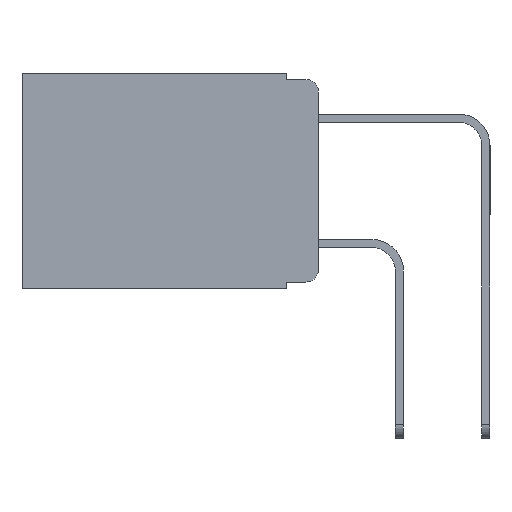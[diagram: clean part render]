
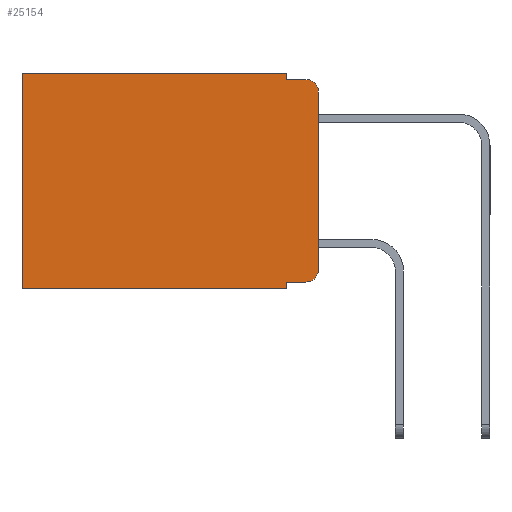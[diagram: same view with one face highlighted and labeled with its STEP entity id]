
A CAD part, left-side view. The second image highlights one B-rep face of the part: STEP entity #25154.
In plain terms, the highlighted planar face has unit normal (-1, 0, 0).
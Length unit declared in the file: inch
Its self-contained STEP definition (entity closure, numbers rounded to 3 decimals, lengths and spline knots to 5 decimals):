
#97 = CARTESIAN_POINT ( 'NONE',  ( 0.298, 0.02, -0.333 ) ) ;
#157 = ORIENTED_EDGE ( 'NONE', *, *, #8219, .T. ) ;
#265 = LINE ( 'NONE', #22726, #15588 ) ;
#322 = DIRECTION ( 'NONE',  ( 0., 0., -1. ) ) ;
#999 = EDGE_CURVE ( 'NONE', #4559, #19389, #6446, .T. ) ;
#1162 = CARTESIAN_POINT ( 'NONE',  ( 0.298, 0.051, 0. ) ) ;
#1246 = DIRECTION ( 'NONE',  ( 0., 0., -1. ) ) ;
#1251 = CARTESIAN_POINT ( 'NONE',  ( 0.298, 0.051, -0.01 ) ) ;
#2074 = VECTOR ( 'NONE', #15118, 39.37008 ) ;
#3204 = CARTESIAN_POINT ( 'NONE',  ( 0.298, 0.473, 0. ) ) ;
#3210 = DIRECTION ( 'NONE',  ( 0., 0., -1. ) ) ;
#3234 = CARTESIAN_POINT ( 'NONE',  ( 0.298, 0., -0.313 ) ) ;
#3296 = DIRECTION ( 'NONE',  ( 0., -1., 0. ) ) ;
#3695 = ORIENTED_EDGE ( 'NONE', *, *, #11364, .F. ) ;
#3890 = ORIENTED_EDGE ( 'NONE', *, *, #19083, .F. ) ;
#4059 = ORIENTED_EDGE ( 'NONE', *, *, #4379, .T. ) ;
#4379 = EDGE_CURVE ( 'NONE', #19259, #4615, #17487, .T. ) ;
#4514 = FACE_OUTER_BOUND ( 'NONE', #5530, .T. ) ;
#4559 = VERTEX_POINT ( 'NONE', #25402 ) ;
#4615 = VERTEX_POINT ( 'NONE', #97 ) ;
#4854 = VERTEX_POINT ( 'NONE', #18906 ) ;
#4895 = VECTOR ( 'NONE', #7200, 39.37008 ) ;
#5078 = CARTESIAN_POINT ( 'NONE',  ( 0.298, 0.051, -0.333 ) ) ;
#5197 = CARTESIAN_POINT ( 'NONE',  ( 0.298, 0., 0. ) ) ;
#5276 = ORIENTED_EDGE ( 'NONE', *, *, #17956, .F. ) ;
#5530 = EDGE_LOOP ( 'NONE', ( #20818, #157, #20794, #3695, #13330, #5594, #5276, #3890, #4059, #6439 ) ) ;
#5594 = ORIENTED_EDGE ( 'NONE', *, *, #6552, .T. ) ;
#5826 = CARTESIAN_POINT ( 'NONE',  ( 0.298, 0.051, 0. ) ) ;
#6439 = ORIENTED_EDGE ( 'NONE', *, *, #10181, .T. ) ;
#6446 = LINE ( 'NONE', #12303, #16381 ) ;
#6552 = EDGE_CURVE ( 'NONE', #4854, #8445, #12056, .T. ) ;
#7068 = DIRECTION ( 'NONE',  ( 0., -1., 0. ) ) ;
#7185 = VECTOR ( 'NONE', #3296, 39.37008 ) ;
#7200 = DIRECTION ( 'NONE',  ( 0., 1., 0. ) ) ;
#8219 = EDGE_CURVE ( 'NONE', #4559, #16452, #25045, .T. ) ;
#8433 = CARTESIAN_POINT ( 'NONE',  ( 0.298, 0.02, -0.03 ) ) ;
#8445 = VERTEX_POINT ( 'NONE', #25031 ) ;
#8740 = CARTESIAN_POINT ( 'NONE',  ( 0.298, 0.051, -0.333 ) ) ;
#10181 = EDGE_CURVE ( 'NONE', #4615, #19389, #19641, .T. ) ;
#10347 = CARTESIAN_POINT ( 'NONE',  ( 0.298, 0.02, -0.313 ) ) ;
#10404 = DIRECTION ( 'NONE',  ( 0., 0., -1. ) ) ;
#11106 = VERTEX_POINT ( 'NONE', #15196 ) ;
#11364 = EDGE_CURVE ( 'NONE', #14459, #25507, #13650, .T. ) ;
#12056 = LINE ( 'NONE', #3204, #2074 ) ;
#12303 = CARTESIAN_POINT ( 'NONE',  ( 0.298, 0., 0. ) ) ;
#12380 = DIRECTION ( 'NONE',  ( 0., 0., -1. ) ) ;
#12963 = AXIS2_PLACEMENT_3D ( 'NONE', #13044, #15127, #3210 ) ;
#13040 = VECTOR ( 'NONE', #1246, 39.37008 ) ;
#13044 = CARTESIAN_POINT ( 'NONE',  ( 0.298, 0., 0. ) ) ;
#13330 = ORIENTED_EDGE ( 'NONE', *, *, #20156, .T. ) ;
#13650 = LINE ( 'NONE', #1162, #13040 ) ;
#14459 = VERTEX_POINT ( 'NONE', #5826 ) ;
#15118 = DIRECTION ( 'NONE',  ( 0., 0., -1. ) ) ;
#15127 = DIRECTION ( 'NONE',  ( 1., 0., 0. ) ) ;
#15196 = CARTESIAN_POINT ( 'NONE',  ( 0.298, 0.051, -0.343 ) ) ;
#15588 = VECTOR ( 'NONE', #22806, 39.37008 ) ;
#16072 = LINE ( 'NONE', #5197, #4895 ) ;
#16381 = VECTOR ( 'NONE', #322, 39.37008 ) ;
#16452 = VERTEX_POINT ( 'NONE', #25714 ) ;
#16521 = AXIS2_PLACEMENT_3D ( 'NONE', #10347, #24308, #12380 ) ;
#17487 = LINE ( 'NONE', #5078, #21562 ) ;
#17775 = LINE ( 'NONE', #1251, #7185 ) ;
#17956 = EDGE_CURVE ( 'NONE', #11106, #8445, #265, .T. ) ;
#18072 = EDGE_CURVE ( 'NONE', #25507, #16452, #17775, .T. ) ;
#18454 = CARTESIAN_POINT ( 'NONE',  ( 0.298, 0.051, -0.01 ) ) ;
#18906 = CARTESIAN_POINT ( 'NONE',  ( 0.298, 0.473, 0. ) ) ;
#19083 = EDGE_CURVE ( 'NONE', #19259, #11106, #19924, .T. ) ;
#19259 = VERTEX_POINT ( 'NONE', #8740 ) ;
#19389 = VERTEX_POINT ( 'NONE', #3234 ) ;
#19641 = CIRCLE ( 'NONE', #16521, 0.02 ) ;
#19924 = LINE ( 'NONE', #22085, #24550 ) ;
#20156 = EDGE_CURVE ( 'NONE', #14459, #4854, #16072, .T. ) ;
#20173 = DIRECTION ( 'NONE',  ( 0., 0., -1. ) ) ;
#20794 = ORIENTED_EDGE ( 'NONE', *, *, #18072, .F. ) ;
#20818 = ORIENTED_EDGE ( 'NONE', *, *, #999, .F. ) ;
#21089 = PLANE ( 'NONE',  #12963 ) ;
#21562 = VECTOR ( 'NONE', #7068, 39.37008 ) ;
#22085 = CARTESIAN_POINT ( 'NONE',  ( 0.298, 0.051, 0. ) ) ;
#22385 = DIRECTION ( 'NONE',  ( -1., 0., 0. ) ) ;
#22726 = CARTESIAN_POINT ( 'NONE',  ( 0.298, 0., -0.343 ) ) ;
#22806 = DIRECTION ( 'NONE',  ( 0., 1., 0. ) ) ;
#24014 = AXIS2_PLACEMENT_3D ( 'NONE', #8433, #22385, #10404 ) ;
#24308 = DIRECTION ( 'NONE',  ( -1., 0., 0. ) ) ;
#24550 = VECTOR ( 'NONE', #20173, 39.37008 ) ;
#25031 = CARTESIAN_POINT ( 'NONE',  ( 0.298, 0.473, -0.343 ) ) ;
#25045 = CIRCLE ( 'NONE', #24014, 0.02 ) ;
#25154 = ADVANCED_FACE ( 'NONE', ( #4514 ), #21089, .F. ) ;
#25402 = CARTESIAN_POINT ( 'NONE',  ( 0.298, 0., -0.03 ) ) ;
#25507 = VERTEX_POINT ( 'NONE', #18454 ) ;
#25714 = CARTESIAN_POINT ( 'NONE',  ( 0.298, 0.02, -0.01 ) ) ;
